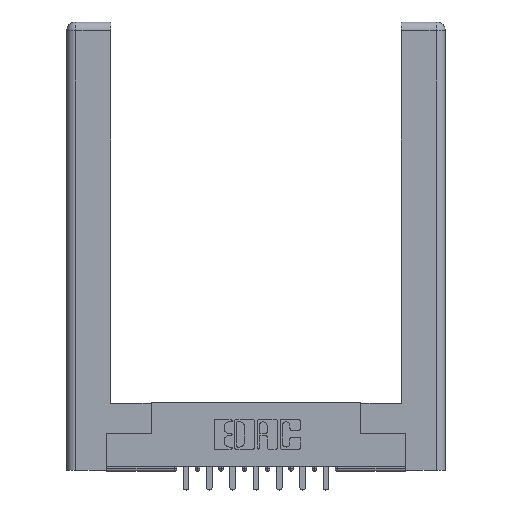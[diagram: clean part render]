
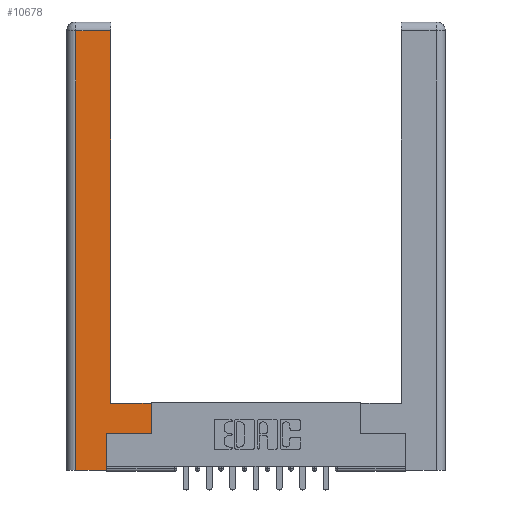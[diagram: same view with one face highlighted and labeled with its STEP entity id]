
A CAD part, top view. The second image highlights one B-rep face of the part: STEP entity #10678.
In plain terms, the highlighted planar face has unit normal (0, 0, 1).
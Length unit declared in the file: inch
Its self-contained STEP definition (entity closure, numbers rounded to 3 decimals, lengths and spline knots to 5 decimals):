
#112 = CARTESIAN_POINT ( 'NONE',  ( 0.0615, 2.94, 0. ) ) ;
#888 = EDGE_CURVE ( 'NONE', #8282, #4651, #10983, .T. ) ;
#1400 = DIRECTION ( 'NONE',  ( -1., 0., 0. ) ) ;
#1488 = CARTESIAN_POINT ( 'NONE',  ( 0.295, 3., 0. ) ) ;
#1543 = ORIENTED_EDGE ( 'NONE', *, *, #7494, .T. ) ;
#1618 = AXIS2_PLACEMENT_3D ( 'NONE', #11564, #2083, #7365 ) ;
#1737 = VERTEX_POINT ( 'NONE', #1872 ) ;
#1792 = LINE ( 'NONE', #3811, #10512 ) ;
#1835 = VECTOR ( 'NONE', #5634, 39.37008 ) ;
#1872 = CARTESIAN_POINT ( 'NONE',  ( 0.265, 0.245, 0. ) ) ;
#2083 = DIRECTION ( 'NONE',  ( 0., 0., -1. ) ) ;
#3062 = CARTESIAN_POINT ( 'NONE',  ( 0.295, 0.45, 0. ) ) ;
#3644 = DIRECTION ( 'NONE',  ( 0., 1., 0. ) ) ;
#3700 = VECTOR ( 'NONE', #5513, 39.37008 ) ;
#3811 = CARTESIAN_POINT ( 'NONE',  ( 0.565, 0.245, 0. ) ) ;
#3825 = EDGE_CURVE ( 'NONE', #1737, #12560, #1792, .T. ) ;
#4143 = VECTOR ( 'NONE', #6851, 39.37008 ) ;
#4315 = EDGE_CURVE ( 'NONE', #6315, #9424, #10814, .T. ) ;
#4510 = CARTESIAN_POINT ( 'NONE',  ( 0.265, 0.245, 0. ) ) ;
#4597 = CARTESIAN_POINT ( 'NONE',  ( 0.565, 0.45, 0. ) ) ;
#4651 = VERTEX_POINT ( 'NONE', #9443 ) ;
#4796 = CARTESIAN_POINT ( 'NONE',  ( 0.565, 0.45, 0. ) ) ;
#4896 = VECTOR ( 'NONE', #1400, 39.37008 ) ;
#5130 = CARTESIAN_POINT ( 'NONE',  ( 0.295, 2.94, 0. ) ) ;
#5356 = LINE ( 'NONE', #4597, #1835 ) ;
#5513 = DIRECTION ( 'NONE',  ( 0., -1., 0. ) ) ;
#5634 = DIRECTION ( 'NONE',  ( 0., 1., 0. ) ) ;
#5650 = ORIENTED_EDGE ( 'NONE', *, *, #13434, .T. ) ;
#5886 = LINE ( 'NONE', #9218, #10942 ) ;
#5968 = CARTESIAN_POINT ( 'NONE',  ( 0.0615, 2.94, 0. ) ) ;
#6061 = VECTOR ( 'NONE', #3644, 39.37008 ) ;
#6098 = VECTOR ( 'NONE', #13162, 39.37008 ) ;
#6315 = VERTEX_POINT ( 'NONE', #5130 ) ;
#6320 = PLANE ( 'NONE',  #1618 ) ;
#6787 = LINE ( 'NONE', #4510, #6098 ) ;
#6851 = DIRECTION ( 'NONE',  ( 1., 0., 0. ) ) ;
#7056 = CARTESIAN_POINT ( 'NONE',  ( 0.265, 0., 0. ) ) ;
#7365 = DIRECTION ( 'NONE',  ( -1., 0., 0. ) ) ;
#7494 = EDGE_CURVE ( 'NONE', #9424, #8282, #9660, .T. ) ;
#7807 = ORIENTED_EDGE ( 'NONE', *, *, #10389, .T. ) ;
#8282 = VERTEX_POINT ( 'NONE', #9494 ) ;
#9015 = DIRECTION ( 'NONE',  ( -1., 0., 0. ) ) ;
#9218 = CARTESIAN_POINT ( 'NONE',  ( 0.295, 0.45, 0. ) ) ;
#9335 = ORIENTED_EDGE ( 'NONE', *, *, #888, .T. ) ;
#9424 = VERTEX_POINT ( 'NONE', #5968 ) ;
#9443 = CARTESIAN_POINT ( 'NONE',  ( 0.265, 0., 0. ) ) ;
#9494 = CARTESIAN_POINT ( 'NONE',  ( 0.0615, 0., 0. ) ) ;
#9660 = LINE ( 'NONE', #11873, #3700 ) ;
#10135 = ORIENTED_EDGE ( 'NONE', *, *, #13388, .T. ) ;
#10173 = DIRECTION ( 'NONE',  ( 1., 0., 0. ) ) ;
#10389 = EDGE_CURVE ( 'NONE', #12560, #13110, #5356, .T. ) ;
#10434 = ORIENTED_EDGE ( 'NONE', *, *, #4315, .T. ) ;
#10512 = VECTOR ( 'NONE', #10173, 39.37008 ) ;
#10678 = ADVANCED_FACE ( 'NONE', ( #13589 ), #6320, .F. ) ;
#10688 = VERTEX_POINT ( 'NONE', #3062 ) ;
#10814 = LINE ( 'NONE', #112, #4896 ) ;
#10942 = VECTOR ( 'NONE', #9015, 39.37008 ) ;
#10983 = LINE ( 'NONE', #7056, #4143 ) ;
#11111 = LINE ( 'NONE', #1488, #6061 ) ;
#11340 = ORIENTED_EDGE ( 'NONE', *, *, #3825, .T. ) ;
#11564 = CARTESIAN_POINT ( 'NONE',  ( 0., 0., 0. ) ) ;
#11730 = EDGE_LOOP ( 'NONE', ( #13427, #10434, #1543, #9335, #10135, #11340, #7807, #5650 ) ) ;
#11873 = CARTESIAN_POINT ( 'NONE',  ( 0.0615, 0., 0. ) ) ;
#11984 = EDGE_CURVE ( 'NONE', #10688, #6315, #11111, .T. ) ;
#12560 = VERTEX_POINT ( 'NONE', #13459 ) ;
#13110 = VERTEX_POINT ( 'NONE', #4796 ) ;
#13162 = DIRECTION ( 'NONE',  ( 0., 1., 0. ) ) ;
#13388 = EDGE_CURVE ( 'NONE', #4651, #1737, #6787, .T. ) ;
#13427 = ORIENTED_EDGE ( 'NONE', *, *, #11984, .T. ) ;
#13434 = EDGE_CURVE ( 'NONE', #13110, #10688, #5886, .T. ) ;
#13459 = CARTESIAN_POINT ( 'NONE',  ( 0.565, 0.245, 0. ) ) ;
#13589 = FACE_OUTER_BOUND ( 'NONE', #11730, .T. ) ;
